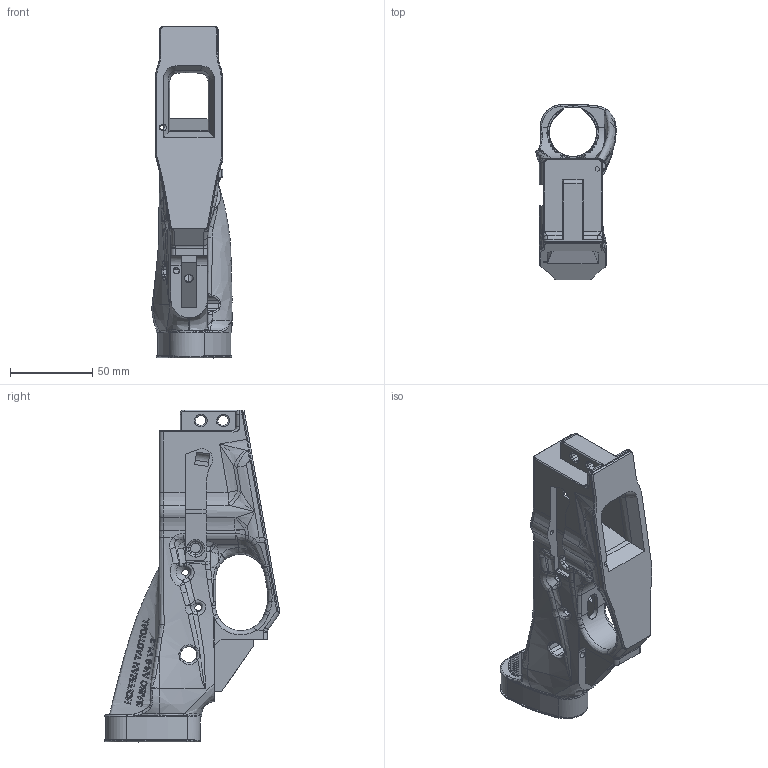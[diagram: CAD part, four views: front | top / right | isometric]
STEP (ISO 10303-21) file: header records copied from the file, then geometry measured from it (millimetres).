
FILE_DESCRIPTION (( 'STEP AP203' ), '1' );
FILE_NAME ('AR-9 BL NS V1.2.STEP', '2022-07-31T19:03:27', ( '' ), ( '' ), 'SwSTEP 2.0', 'SolidWorks 2021', '' );
FILE_SCHEMA (( 'CONFIG_CONTROL_DESIGN' ));
Products named in the file (1): AR-9 BL NS V1.2
Bounding box: 48.72 x 106.75 x 201.55 mm (x, y, z)
Volume: 215705.7 mm3; surface area: 64836.3 mm2
Topology: 1 solids, 1 shells, 1702 faces, 4558 edges, 2886 vertices
Faces by surface type: bspline 1019, plane 305, cylinder 271, torus 60, cone 34, sphere 13
Entity records: 242075 total; most frequent: CARTESIAN_POINT 208477, ORIENTED_EDGE 9040, EDGE_CURVE 4520, DIRECTION 3808, VERTEX_POINT 2886, B_SPLINE_CURVE_WITH_KNOTS 2426, EDGE_LOOP 1810, ADVANCED_FACE 1702
